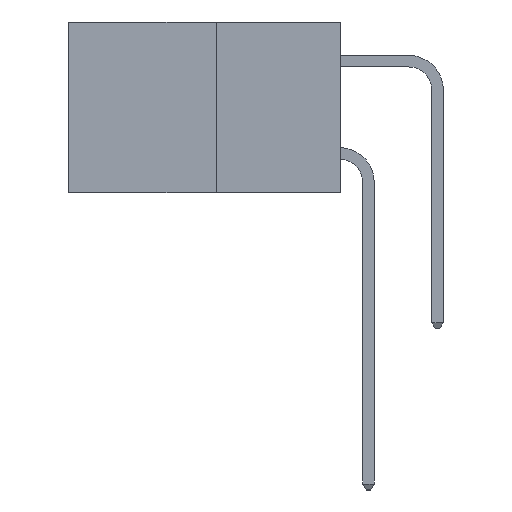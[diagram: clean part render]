
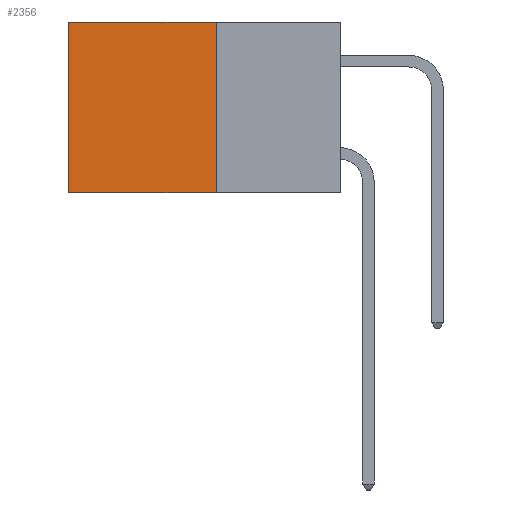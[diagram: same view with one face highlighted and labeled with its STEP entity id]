
A CAD part, left-side view. The second image highlights one B-rep face of the part: STEP entity #2356.
In plain terms, the highlighted planar face has unit normal (-1, 0, 0).
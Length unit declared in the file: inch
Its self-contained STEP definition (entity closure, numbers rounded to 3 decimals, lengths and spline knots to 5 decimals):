
#307 = VECTOR ( 'NONE', #12270, 39.37008 ) ;
#374 = EDGE_CURVE ( 'NONE', #2857, #1990, #10604, .T. ) ;
#1112 = CARTESIAN_POINT ( 'NONE',  ( 0.277, 0.59, -0.37 ) ) ;
#1624 = CARTESIAN_POINT ( 'NONE',  ( 0.277, 0.59, -0.37 ) ) ;
#1752 = EDGE_CURVE ( 'NONE', #1990, #11332, #2927, .T. ) ;
#1758 = CARTESIAN_POINT ( 'NONE',  ( 0.277, 0.27, 0. ) ) ;
#1970 = ORIENTED_EDGE ( 'NONE', *, *, #1752, .T. ) ;
#1990 = VERTEX_POINT ( 'NONE', #10867 ) ;
#2356 = ADVANCED_FACE ( 'NONE', ( #4180 ), #2910, .F. ) ;
#2467 = EDGE_CURVE ( 'NONE', #12048, #11332, #8061, .T. ) ;
#2504 = EDGE_LOOP ( 'NONE', ( #1970, #7178, #2575, #8344 ) ) ;
#2575 = ORIENTED_EDGE ( 'NONE', *, *, #5529, .F. ) ;
#2795 = CARTESIAN_POINT ( 'NONE',  ( 0.277, 0.27, -0.37 ) ) ;
#2837 = DIRECTION ( 'NONE',  ( 1., 0., 0. ) ) ;
#2853 = DIRECTION ( 'NONE',  ( 0., 0., -1. ) ) ;
#2857 = VERTEX_POINT ( 'NONE', #1758 ) ;
#2910 = PLANE ( 'NONE',  #4544 ) ;
#2927 = LINE ( 'NONE', #1112, #307 ) ;
#3369 = LINE ( 'NONE', #7628, #10706 ) ;
#4180 = FACE_OUTER_BOUND ( 'NONE', #2504, .T. ) ;
#4544 = AXIS2_PLACEMENT_3D ( 'NONE', #2795, #2837, #2853 ) ;
#5300 = VECTOR ( 'NONE', #11660, 39.37008 ) ;
#5529 = EDGE_CURVE ( 'NONE', #2857, #12048, #3369, .T. ) ;
#7178 = ORIENTED_EDGE ( 'NONE', *, *, #2467, .F. ) ;
#7628 = CARTESIAN_POINT ( 'NONE',  ( 0.277, 0.27, -0.37 ) ) ;
#8061 = LINE ( 'NONE', #10410, #8375 ) ;
#8344 = ORIENTED_EDGE ( 'NONE', *, *, #374, .T. ) ;
#8375 = VECTOR ( 'NONE', #10650, 39.37008 ) ;
#8862 = DIRECTION ( 'NONE',  ( 0., 0., -1. ) ) ;
#10410 = CARTESIAN_POINT ( 'NONE',  ( 0.277, 0.27, -0.37 ) ) ;
#10604 = LINE ( 'NONE', #12083, #5300 ) ;
#10650 = DIRECTION ( 'NONE',  ( 0., 1., 0. ) ) ;
#10706 = VECTOR ( 'NONE', #8862, 39.37008 ) ;
#10867 = CARTESIAN_POINT ( 'NONE',  ( 0.277, 0.59, 0. ) ) ;
#11332 = VERTEX_POINT ( 'NONE', #1624 ) ;
#11513 = CARTESIAN_POINT ( 'NONE',  ( 0.277, 0.27, -0.37 ) ) ;
#11660 = DIRECTION ( 'NONE',  ( 0., 1., 0. ) ) ;
#12048 = VERTEX_POINT ( 'NONE', #11513 ) ;
#12083 = CARTESIAN_POINT ( 'NONE',  ( 0.277, 0.27, 0. ) ) ;
#12270 = DIRECTION ( 'NONE',  ( 0., 0., -1. ) ) ;
